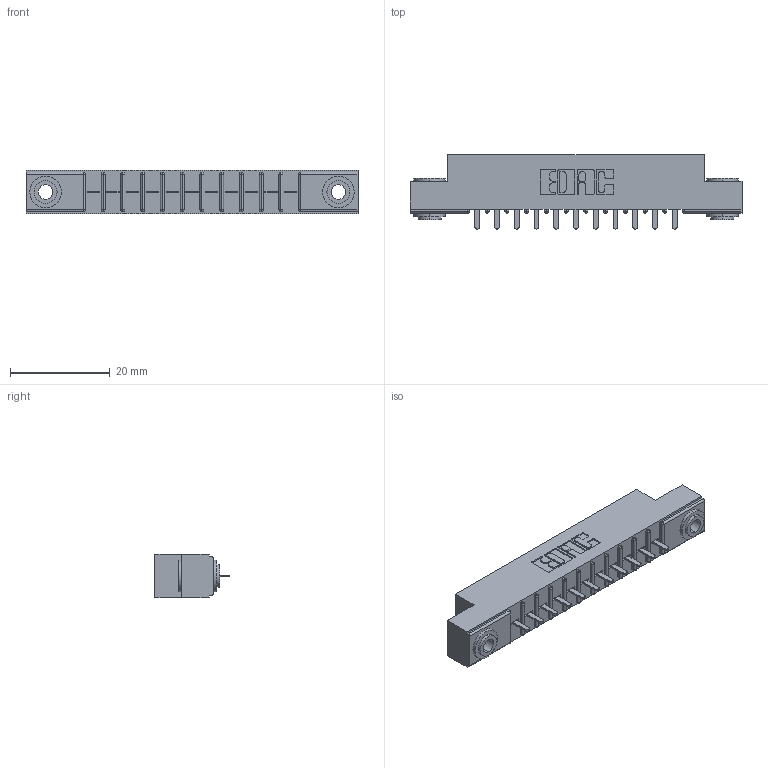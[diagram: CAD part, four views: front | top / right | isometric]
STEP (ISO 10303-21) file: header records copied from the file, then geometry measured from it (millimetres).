
FILE_DESCRIPTION (( 'STEP AP203' ), '1' );
FILE_NAME ('316-011-521-103.STEP', '2018-07-31T00:18:54', ( '' ), ( '' ), 'SwSTEP 2.0', 'SolidWorks 2016', '' );
FILE_SCHEMA (( 'CONFIG_CONTROL_DESIGN' ));
Length unit declared in the file: inch
Products named in the file (4): 306 Part_.156 Dia; 306-290-001_121; 345-250-002_345-250-002-102; 316-011-521-103
Assembly tree (14 placements, depth 2):
  316-011-521-103
    306 Part_.156 Dia
    306-290-001_121  x11
    345-250-002_345-250-002-102  x2
Bounding box: 66.6 x 14.88 x 8.71 mm (x, y, z)
Volume: 4497.4 mm3; surface area: 6469.8 mm2
Topology: 14 solids, 14 shells, 938 faces, 2595 edges, 1666 vertices
Faces by surface type: plane 609, cylinder 277, sphere 44, cone 8
Entity records: 15295 total; most frequent: CARTESIAN_POINT 2541, DIRECTION 2523, ORIENTED_EDGE 2506, EDGE_CURVE 1253, VECTOR 955, LINE 955, VERTEX_POINT 802, AXIS2_PLACEMENT_3D 784
